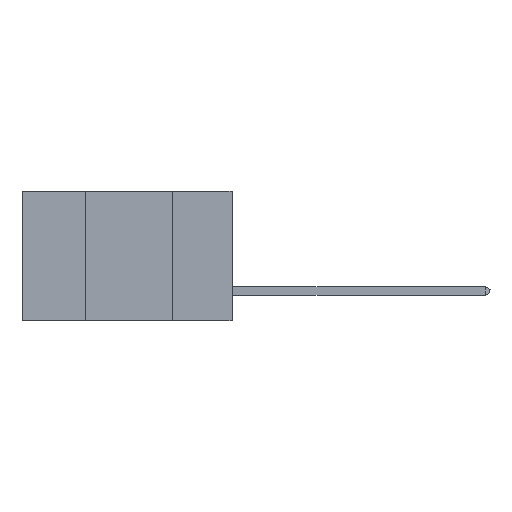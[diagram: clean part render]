
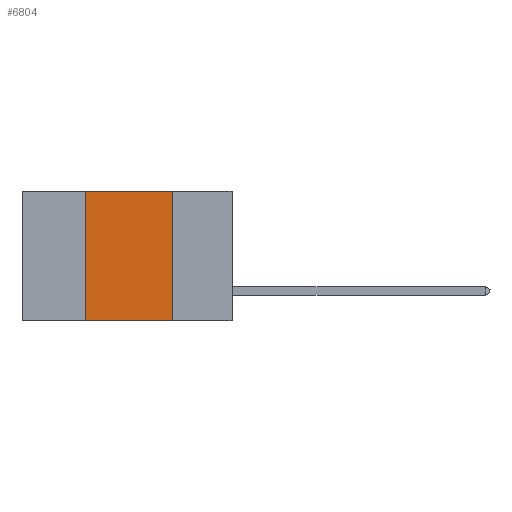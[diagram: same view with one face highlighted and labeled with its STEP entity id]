
A CAD part, left-side view. The second image highlights one B-rep face of the part: STEP entity #6804.
In plain terms, the highlighted planar face has unit normal (-1, 0, 0).
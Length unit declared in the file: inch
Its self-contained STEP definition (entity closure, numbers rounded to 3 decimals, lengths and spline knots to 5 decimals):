
#22 = VERTEX_POINT ( 'NONE', #5217 ) ;
#151 = ORIENTED_EDGE ( 'NONE', *, *, #5385, .F. ) ;
#210 = CARTESIAN_POINT ( 'NONE',  ( 0., 0.17, -0.37 ) ) ;
#1360 = EDGE_LOOP ( 'NONE', ( #151, #3206, #11071, #7921 ) ) ;
#1699 = EDGE_CURVE ( 'NONE', #17524, #22, #8589, .T. ) ;
#1960 = VECTOR ( 'NONE', #19315, 39.37008 ) ;
#2469 = PLANE ( 'NONE',  #8818 ) ;
#2592 = VECTOR ( 'NONE', #9303, 39.37008 ) ;
#2629 = EDGE_CURVE ( 'NONE', #5233, #17524, #12125, .T. ) ;
#2958 = VECTOR ( 'NONE', #6853, 39.37008 ) ;
#3033 = CARTESIAN_POINT ( 'NONE',  ( 0., 0.6, -0.37 ) ) ;
#3206 = ORIENTED_EDGE ( 'NONE', *, *, #1699, .F. ) ;
#4033 = DIRECTION ( 'NONE',  ( 0., 0., -1. ) ) ;
#5115 = CARTESIAN_POINT ( 'NONE',  ( 0., 0.42, -0.37 ) ) ;
#5217 = CARTESIAN_POINT ( 'NONE',  ( 0., 0.17, 0. ) ) ;
#5233 = VERTEX_POINT ( 'NONE', #5115 ) ;
#5257 = LINE ( 'NONE', #3033, #2592 ) ;
#5385 = EDGE_CURVE ( 'NONE', #22, #13141, #6983, .T. ) ;
#6804 = ADVANCED_FACE ( 'NONE', ( #16988 ), #2469, .F. ) ;
#6853 = DIRECTION ( 'NONE',  ( 0., 0., 1. ) ) ;
#6983 = LINE ( 'NONE', #14460, #9604 ) ;
#7921 = ORIENTED_EDGE ( 'NONE', *, *, #17479, .T. ) ;
#8589 = LINE ( 'NONE', #19255, #1960 ) ;
#8818 = AXIS2_PLACEMENT_3D ( 'NONE', #16528, #18010, #4033 ) ;
#9303 = DIRECTION ( 'NONE',  ( 0., -1., 0. ) ) ;
#9604 = VECTOR ( 'NONE', #14254, 39.37008 ) ;
#11071 = ORIENTED_EDGE ( 'NONE', *, *, #2629, .F. ) ;
#12125 = LINE ( 'NONE', #14564, #2958 ) ;
#13141 = VERTEX_POINT ( 'NONE', #210 ) ;
#14254 = DIRECTION ( 'NONE',  ( 0., 0., -1. ) ) ;
#14460 = CARTESIAN_POINT ( 'NONE',  ( 0., 0.17, 0. ) ) ;
#14564 = CARTESIAN_POINT ( 'NONE',  ( 0., 0.42, 0. ) ) ;
#16528 = CARTESIAN_POINT ( 'NONE',  ( 0., 0.6, 0. ) ) ;
#16988 = FACE_OUTER_BOUND ( 'NONE', #1360, .T. ) ;
#17099 = CARTESIAN_POINT ( 'NONE',  ( 0., 0.42, 0. ) ) ;
#17479 = EDGE_CURVE ( 'NONE', #5233, #13141, #5257, .T. ) ;
#17524 = VERTEX_POINT ( 'NONE', #17099 ) ;
#18010 = DIRECTION ( 'NONE',  ( 1., 0., 0. ) ) ;
#19255 = CARTESIAN_POINT ( 'NONE',  ( 0., 0.6, 0. ) ) ;
#19315 = DIRECTION ( 'NONE',  ( 0., -1., 0. ) ) ;
